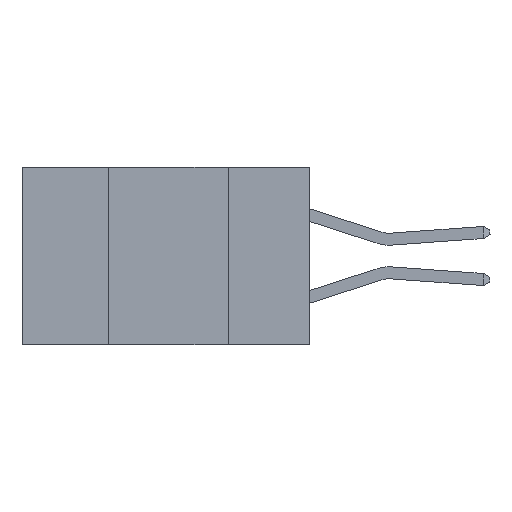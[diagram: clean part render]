
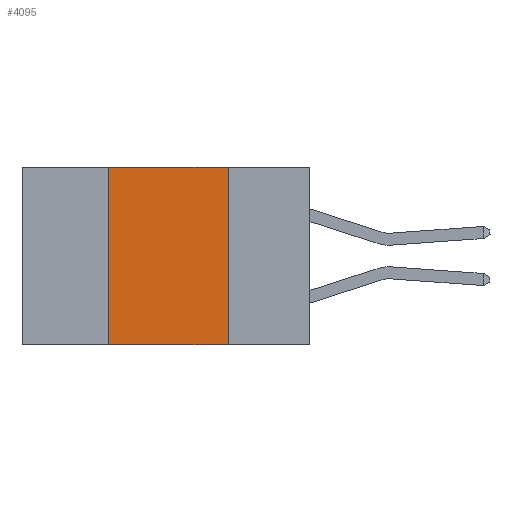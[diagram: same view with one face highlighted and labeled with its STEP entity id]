
A CAD part, left-side view. The second image highlights one B-rep face of the part: STEP entity #4095.
In plain terms, the highlighted planar face has unit normal (-1, 0, 0).
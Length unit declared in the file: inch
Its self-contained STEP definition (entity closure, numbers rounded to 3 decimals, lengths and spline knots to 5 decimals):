
#489 = ORIENTED_EDGE ( 'NONE', *, *, #13083, .F. ) ;
#1456 = ORIENTED_EDGE ( 'NONE', *, *, #17408, .F. ) ;
#3134 = VECTOR ( 'NONE', #3880, 39.37008 ) ;
#3860 = LINE ( 'NONE', #21416, #25284 ) ;
#3880 = DIRECTION ( 'NONE',  ( 0., 0., 1. ) ) ;
#4095 = ADVANCED_FACE ( 'NONE', ( #18797 ), #13134, .F. ) ;
#4556 = EDGE_CURVE ( 'NONE', #8527, #22846, #15086, .T. ) ;
#4663 = VECTOR ( 'NONE', #8636, 39.37008 ) ;
#5064 = VERTEX_POINT ( 'NONE', #18512 ) ;
#6537 = CARTESIAN_POINT ( 'NONE',  ( 0., 0.17, 0. ) ) ;
#8527 = VERTEX_POINT ( 'NONE', #19897 ) ;
#8636 = DIRECTION ( 'NONE',  ( 0., 0., -1. ) ) ;
#8696 = LINE ( 'NONE', #20419, #3134 ) ;
#10648 = ORIENTED_EDGE ( 'NONE', *, *, #4556, .T. ) ;
#10829 = DIRECTION ( 'NONE',  ( 0., -1., 0. ) ) ;
#11090 = DIRECTION ( 'NONE',  ( 0., -1., 0. ) ) ;
#11129 = DIRECTION ( 'NONE',  ( 1., 0., 0. ) ) ;
#12284 = EDGE_LOOP ( 'NONE', ( #1456, #24212, #489, #10648 ) ) ;
#13083 = EDGE_CURVE ( 'NONE', #8527, #5064, #8696, .T. ) ;
#13134 = PLANE ( 'NONE',  #21064 ) ;
#15086 = LINE ( 'NONE', #23220, #19962 ) ;
#15745 = LINE ( 'NONE', #6537, #4663 ) ;
#17285 = CARTESIAN_POINT ( 'NONE',  ( 0., 0.6, 0. ) ) ;
#17408 = EDGE_CURVE ( 'NONE', #20105, #22846, #15745, .T. ) ;
#18140 = CARTESIAN_POINT ( 'NONE',  ( 0., 0.17, 0. ) ) ;
#18512 = CARTESIAN_POINT ( 'NONE',  ( 0., 0.42, 0. ) ) ;
#18797 = FACE_OUTER_BOUND ( 'NONE', #12284, .T. ) ;
#19897 = CARTESIAN_POINT ( 'NONE',  ( 0., 0.42, -0.37 ) ) ;
#19962 = VECTOR ( 'NONE', #10829, 39.37008 ) ;
#20105 = VERTEX_POINT ( 'NONE', #18140 ) ;
#20419 = CARTESIAN_POINT ( 'NONE',  ( 0., 0.42, 0. ) ) ;
#21064 = AXIS2_PLACEMENT_3D ( 'NONE', #17285, #11129, #25593 ) ;
#21416 = CARTESIAN_POINT ( 'NONE',  ( 0., 0.6, 0. ) ) ;
#22846 = VERTEX_POINT ( 'NONE', #24251 ) ;
#23220 = CARTESIAN_POINT ( 'NONE',  ( 0., 0.6, -0.37 ) ) ;
#24212 = ORIENTED_EDGE ( 'NONE', *, *, #26609, .F. ) ;
#24251 = CARTESIAN_POINT ( 'NONE',  ( 0., 0.17, -0.37 ) ) ;
#25284 = VECTOR ( 'NONE', #11090, 39.37008 ) ;
#25593 = DIRECTION ( 'NONE',  ( 0., 0., -1. ) ) ;
#26609 = EDGE_CURVE ( 'NONE', #5064, #20105, #3860, .T. ) ;
